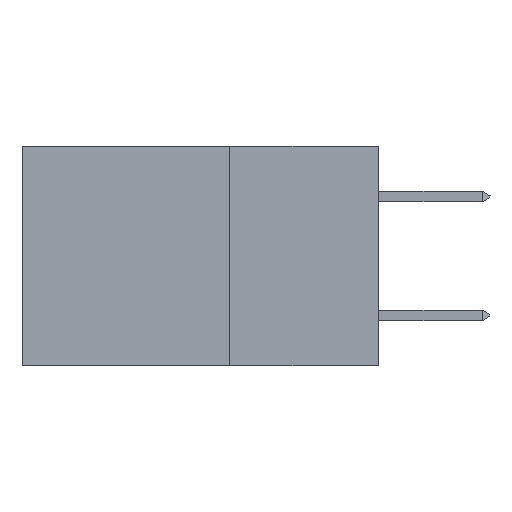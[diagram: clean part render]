
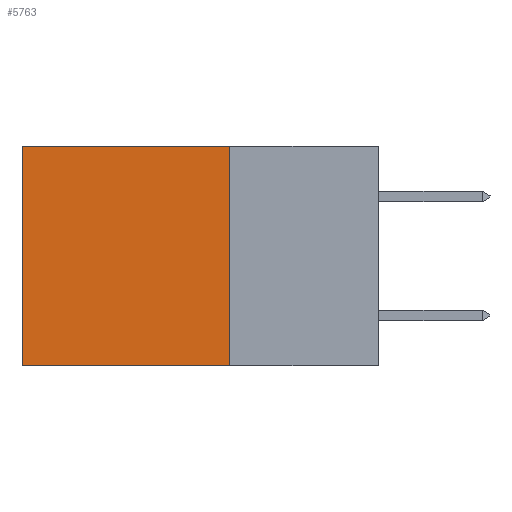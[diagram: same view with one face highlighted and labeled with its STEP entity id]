
A CAD part, left-side view. The second image highlights one B-rep face of the part: STEP entity #5763.
In plain terms, the highlighted planar face has unit normal (-1, 0, 0).
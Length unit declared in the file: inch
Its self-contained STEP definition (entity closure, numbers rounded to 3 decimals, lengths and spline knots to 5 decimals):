
#398 = ORIENTED_EDGE ( 'NONE', *, *, #9301, .T. ) ;
#829 = CARTESIAN_POINT ( 'NONE',  ( 0.2615, 0.25, 0. ) ) ;
#877 = VECTOR ( 'NONE', #1845, 39.37008 ) ;
#1845 = DIRECTION ( 'NONE',  ( 0., 0., -1. ) ) ;
#1985 = DIRECTION ( 'NONE',  ( 0., 1., 0. ) ) ;
#2171 = VECTOR ( 'NONE', #9113, 39.37008 ) ;
#2454 = DIRECTION ( 'NONE',  ( 1., 0., 0. ) ) ;
#2474 = DIRECTION ( 'NONE',  ( 0., 1., 0. ) ) ;
#3140 = VERTEX_POINT ( 'NONE', #12528 ) ;
#3402 = CARTESIAN_POINT ( 'NONE',  ( 0.2615, 0.6, -0.37 ) ) ;
#3636 = LINE ( 'NONE', #5820, #6881 ) ;
#3763 = EDGE_CURVE ( 'NONE', #3140, #6035, #3636, .T. ) ;
#4468 = CARTESIAN_POINT ( 'NONE',  ( 0.2615, 0.6, 0. ) ) ;
#4579 = FACE_OUTER_BOUND ( 'NONE', #6100, .T. ) ;
#5062 = CARTESIAN_POINT ( 'NONE',  ( 0.2615, 0.6, -0.37 ) ) ;
#5065 = LINE ( 'NONE', #829, #5398 ) ;
#5302 = CARTESIAN_POINT ( 'NONE',  ( 0.2615, 0.25, 0. ) ) ;
#5351 = EDGE_CURVE ( 'NONE', #10410, #6035, #10383, .T. ) ;
#5398 = VECTOR ( 'NONE', #1985, 39.37008 ) ;
#5763 = ADVANCED_FACE ( 'NONE', ( #4579 ), #11774, .F. ) ;
#5820 = CARTESIAN_POINT ( 'NONE',  ( 0.2615, 0.25, -0.37 ) ) ;
#5965 = CARTESIAN_POINT ( 'NONE',  ( 0.2615, 0.25, -0.37 ) ) ;
#6035 = VERTEX_POINT ( 'NONE', #3402 ) ;
#6100 = EDGE_LOOP ( 'NONE', ( #6444, #8460, #10273, #398 ) ) ;
#6444 = ORIENTED_EDGE ( 'NONE', *, *, #5351, .T. ) ;
#6635 = DIRECTION ( 'NONE',  ( 0., 0., -1. ) ) ;
#6830 = CARTESIAN_POINT ( 'NONE',  ( 0.2615, 0.25, -0.37 ) ) ;
#6881 = VECTOR ( 'NONE', #2474, 39.37008 ) ;
#8437 = VERTEX_POINT ( 'NONE', #5302 ) ;
#8460 = ORIENTED_EDGE ( 'NONE', *, *, #3763, .F. ) ;
#9113 = DIRECTION ( 'NONE',  ( 0., 0., -1. ) ) ;
#9301 = EDGE_CURVE ( 'NONE', #8437, #10410, #5065, .T. ) ;
#10273 = ORIENTED_EDGE ( 'NONE', *, *, #11903, .F. ) ;
#10383 = LINE ( 'NONE', #5062, #877 ) ;
#10410 = VERTEX_POINT ( 'NONE', #4468 ) ;
#10979 = AXIS2_PLACEMENT_3D ( 'NONE', #6830, #2454, #6635 ) ;
#11127 = LINE ( 'NONE', #5965, #2171 ) ;
#11774 = PLANE ( 'NONE',  #10979 ) ;
#11903 = EDGE_CURVE ( 'NONE', #8437, #3140, #11127, .T. ) ;
#12528 = CARTESIAN_POINT ( 'NONE',  ( 0.2615, 0.25, -0.37 ) ) ;
